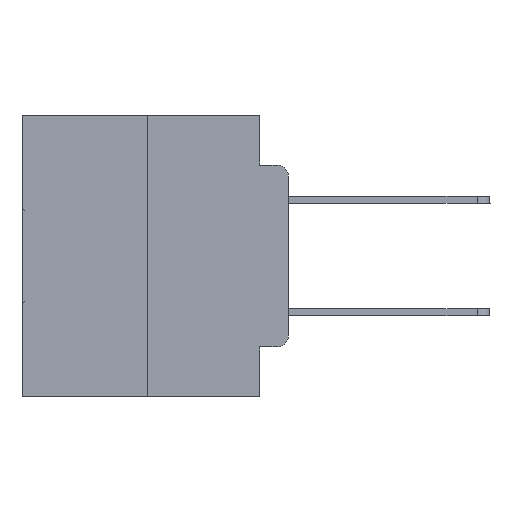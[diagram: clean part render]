
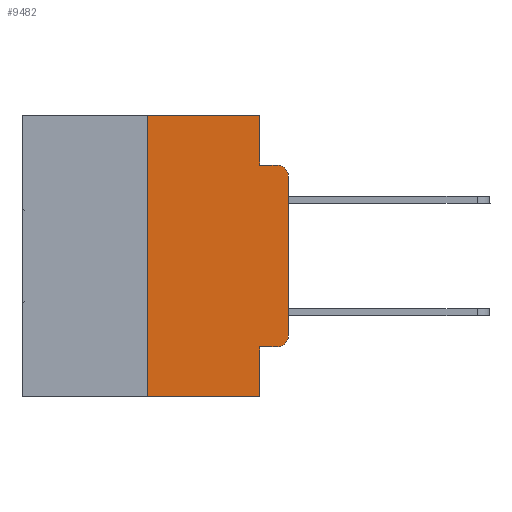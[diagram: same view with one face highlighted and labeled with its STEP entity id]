
A CAD part, left-side view. The second image highlights one B-rep face of the part: STEP entity #9482.
In plain terms, the highlighted planar face has unit normal (-1, 0, 0).
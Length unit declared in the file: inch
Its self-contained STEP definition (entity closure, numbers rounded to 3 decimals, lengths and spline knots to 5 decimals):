
#157 = ORIENTED_EDGE ( 'NONE', *, *, #16077, .T. ) ;
#712 = ORIENTED_EDGE ( 'NONE', *, *, #21564, .T. ) ;
#763 = LINE ( 'NONE', #28476, #9303 ) ;
#915 = EDGE_CURVE ( 'NONE', #27035, #16127, #8963, .T. ) ;
#1104 = ORIENTED_EDGE ( 'NONE', *, *, #24677, .T. ) ;
#1421 = VERTEX_POINT ( 'NONE', #31561 ) ;
#1497 = VECTOR ( 'NONE', #26795, 39.37008 ) ;
#1743 = EDGE_CURVE ( 'NONE', #24598, #27035, #763, .T. ) ;
#2771 = VECTOR ( 'NONE', #31085, 39.37008 ) ;
#2826 = CARTESIAN_POINT ( 'NONE',  ( 0., 0.25, -0.5 ) ) ;
#2878 = ORIENTED_EDGE ( 'NONE', *, *, #19144, .F. ) ;
#3217 = LINE ( 'NONE', #31715, #18844 ) ;
#3424 = EDGE_CURVE ( 'NONE', #18414, #16548, #29400, .T. ) ;
#3510 = CARTESIAN_POINT ( 'NONE',  ( 0., 0.051, -0.5 ) ) ;
#4646 = CARTESIAN_POINT ( 'NONE',  ( 0., 0.473, -0.5 ) ) ;
#5721 = CARTESIAN_POINT ( 'NONE',  ( 0., 0.051, -0.4115 ) ) ;
#6279 = EDGE_CURVE ( 'NONE', #25943, #31141, #24120, .T. ) ;
#6741 = DIRECTION ( 'NONE',  ( 0., 0., -1. ) ) ;
#7008 = ORIENTED_EDGE ( 'NONE', *, *, #915, .F. ) ;
#7042 = CIRCLE ( 'NONE', #20342, 0.02 ) ;
#7877 = LINE ( 'NONE', #18677, #11852 ) ;
#8021 = ORIENTED_EDGE ( 'NONE', *, *, #1743, .F. ) ;
#8625 = CARTESIAN_POINT ( 'NONE',  ( 0., 0.02, -0.4115 ) ) ;
#8821 = DIRECTION ( 'NONE',  ( 0., 0., 1. ) ) ;
#8857 = DIRECTION ( 'NONE',  ( -1., 0., 0. ) ) ;
#8862 = CARTESIAN_POINT ( 'NONE',  ( 0., 0.051, 0. ) ) ;
#8963 = LINE ( 'NONE', #30977, #2771 ) ;
#9303 = VECTOR ( 'NONE', #26147, 39.37008 ) ;
#9393 = DIRECTION ( 'NONE',  ( 0., -1., 0. ) ) ;
#9482 = ADVANCED_FACE ( 'NONE', ( #19816 ), #32359, .F. ) ;
#9711 = CARTESIAN_POINT ( 'NONE',  ( 0., 0.25, 0. ) ) ;
#11327 = VECTOR ( 'NONE', #30803, 39.37008 ) ;
#11496 = DIRECTION ( 'NONE',  ( 0., 0., -1. ) ) ;
#11852 = VECTOR ( 'NONE', #8821, 39.37008 ) ;
#11903 = AXIS2_PLACEMENT_3D ( 'NONE', #27506, #17333, #12201 ) ;
#12201 = DIRECTION ( 'NONE',  ( 0., 0., -1. ) ) ;
#12317 = CARTESIAN_POINT ( 'NONE',  ( 0., 0., -0.1085 ) ) ;
#15621 = EDGE_CURVE ( 'NONE', #25943, #25040, #26943, .T. ) ;
#15946 = CARTESIAN_POINT ( 'NONE',  ( 0., 0.051, -0.4115 ) ) ;
#16077 = EDGE_CURVE ( 'NONE', #24136, #16127, #23339, .T. ) ;
#16127 = VERTEX_POINT ( 'NONE', #17199 ) ;
#16548 = VERTEX_POINT ( 'NONE', #8625 ) ;
#16648 = DIRECTION ( 'NONE',  ( -1., 0., 0. ) ) ;
#17199 = CARTESIAN_POINT ( 'NONE',  ( 0., 0.02, -0.0885 ) ) ;
#17333 = DIRECTION ( 'NONE',  ( 1., 0., 0. ) ) ;
#17966 = LINE ( 'NONE', #18190, #11327 ) ;
#18190 = CARTESIAN_POINT ( 'NONE',  ( 0., 0.473, 0. ) ) ;
#18414 = VERTEX_POINT ( 'NONE', #15946 ) ;
#18677 = CARTESIAN_POINT ( 'NONE',  ( 0., 0., 0. ) ) ;
#18844 = VECTOR ( 'NONE', #6741, 39.37008 ) ;
#19144 = EDGE_CURVE ( 'NONE', #18414, #25040, #3217, .T. ) ;
#19423 = CARTESIAN_POINT ( 'NONE',  ( 0., 0.02, -0.3915 ) ) ;
#19816 = FACE_OUTER_BOUND ( 'NONE', #28046, .T. ) ;
#20342 = AXIS2_PLACEMENT_3D ( 'NONE', #19423, #16648, #29254 ) ;
#20803 = DIRECTION ( 'NONE',  ( 0., -1., 0. ) ) ;
#21035 = VECTOR ( 'NONE', #9393, 39.37008 ) ;
#21108 = VECTOR ( 'NONE', #20803, 39.37008 ) ;
#21564 = EDGE_CURVE ( 'NONE', #1421, #24136, #7877, .T. ) ;
#23339 = CIRCLE ( 'NONE', #25596, 0.02 ) ;
#23563 = EDGE_CURVE ( 'NONE', #31141, #24598, #17966, .T. ) ;
#24120 = LINE ( 'NONE', #9711, #1497 ) ;
#24136 = VERTEX_POINT ( 'NONE', #12317 ) ;
#24598 = VERTEX_POINT ( 'NONE', #8862 ) ;
#24677 = EDGE_CURVE ( 'NONE', #16548, #1421, #7042, .T. ) ;
#25040 = VERTEX_POINT ( 'NONE', #3510 ) ;
#25596 = AXIS2_PLACEMENT_3D ( 'NONE', #31684, #8857, #11496 ) ;
#25683 = ORIENTED_EDGE ( 'NONE', *, *, #3424, .T. ) ;
#25693 = ORIENTED_EDGE ( 'NONE', *, *, #15621, .T. ) ;
#25943 = VERTEX_POINT ( 'NONE', #2826 ) ;
#26142 = ORIENTED_EDGE ( 'NONE', *, *, #23563, .F. ) ;
#26147 = DIRECTION ( 'NONE',  ( 0., 0., -1. ) ) ;
#26795 = DIRECTION ( 'NONE',  ( 0., 0., 1. ) ) ;
#26943 = LINE ( 'NONE', #4646, #21035 ) ;
#27035 = VERTEX_POINT ( 'NONE', #29556 ) ;
#27506 = CARTESIAN_POINT ( 'NONE',  ( 0., 0.473, 0. ) ) ;
#28046 = EDGE_LOOP ( 'NONE', ( #712, #157, #7008, #8021, #26142, #29055, #25693, #2878, #25683, #1104 ) ) ;
#28476 = CARTESIAN_POINT ( 'NONE',  ( 0., 0.051, 0. ) ) ;
#29055 = ORIENTED_EDGE ( 'NONE', *, *, #6279, .F. ) ;
#29254 = DIRECTION ( 'NONE',  ( 0., 0., -1. ) ) ;
#29400 = LINE ( 'NONE', #5721, #21108 ) ;
#29556 = CARTESIAN_POINT ( 'NONE',  ( 0., 0.051, -0.0885 ) ) ;
#30803 = DIRECTION ( 'NONE',  ( 0., -1., 0. ) ) ;
#30977 = CARTESIAN_POINT ( 'NONE',  ( 0., 0.051, -0.0885 ) ) ;
#31085 = DIRECTION ( 'NONE',  ( 0., -1., 0. ) ) ;
#31141 = VERTEX_POINT ( 'NONE', #31782 ) ;
#31561 = CARTESIAN_POINT ( 'NONE',  ( 0., 0., -0.3915 ) ) ;
#31684 = CARTESIAN_POINT ( 'NONE',  ( 0., 0.02, -0.1085 ) ) ;
#31715 = CARTESIAN_POINT ( 'NONE',  ( 0., 0.051, 0. ) ) ;
#31782 = CARTESIAN_POINT ( 'NONE',  ( 0., 0.25, 0. ) ) ;
#32359 = PLANE ( 'NONE',  #11903 ) ;
